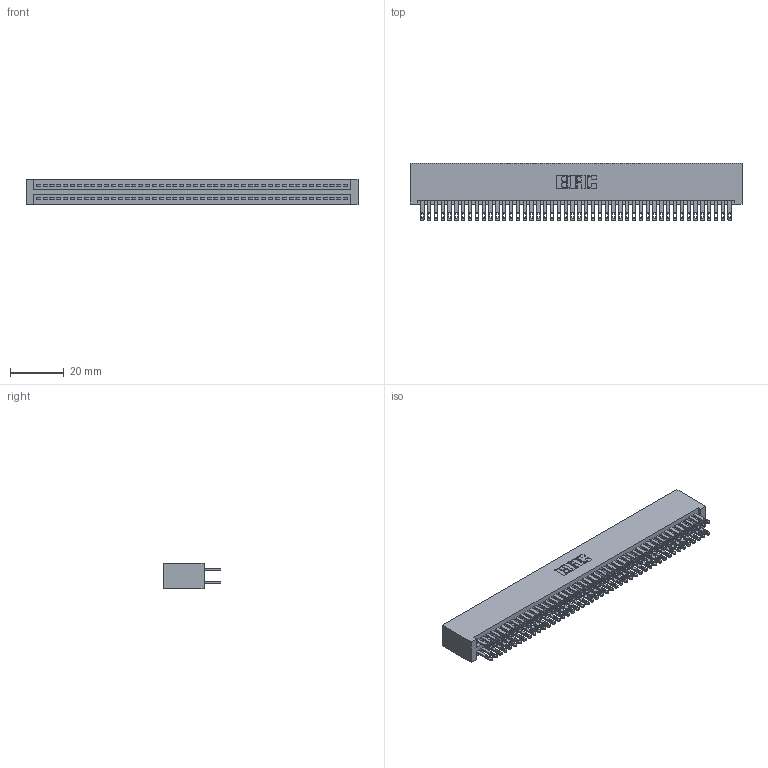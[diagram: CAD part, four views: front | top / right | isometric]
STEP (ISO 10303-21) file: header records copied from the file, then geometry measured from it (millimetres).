
FILE_DESCRIPTION (( 'STEP AP203' ), '1' );
FILE_NAME ('345-092-500-201.STEP', '2019-11-01T17:53:28', ( '' ), ( '' ), 'SwSTEP 2.0', 'SolidWorks 2016', '' );
FILE_SCHEMA (( 'CONFIG_CONTROL_DESIGN' ));
Length unit declared in the file: inch
Products named in the file (3): 345-292-001_345-293-100; 345 Part_No Mounting Lugs; 345-092-500-201
Assembly tree (93 placements, depth 2):
  345-092-500-201
    345 Part_No Mounting Lugs
    345-292-001_345-293-100  x92
Bounding box: 123.44 x 21.51 x 9.4 mm (x, y, z)
Volume: 12925.7 mm3; surface area: 20425.4 mm2
Topology: 93 solids, 93 shells, 4350 faces, 13289 edges, 8858 vertices
Faces by surface type: plane 2560, cylinder 1790
Entity records: 35207 total; most frequent: CARTESIAN_POINT 5896, ORIENTED_EDGE 5830, DIRECTION 5191, EDGE_CURVE 2915, VECTOR 2603, LINE 2603, VERTEX_POINT 1942, AXIS2_PLACEMENT_3D 1294
